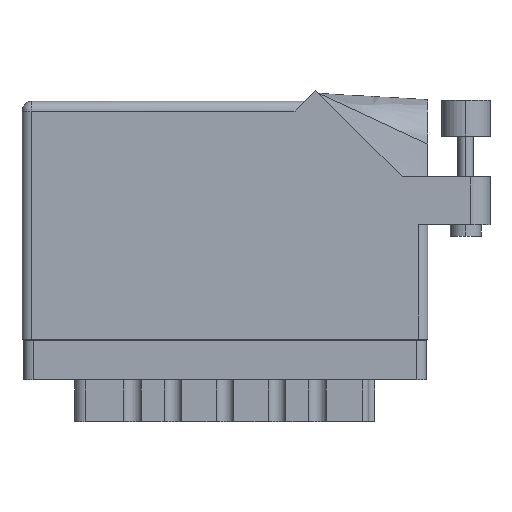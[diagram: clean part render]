
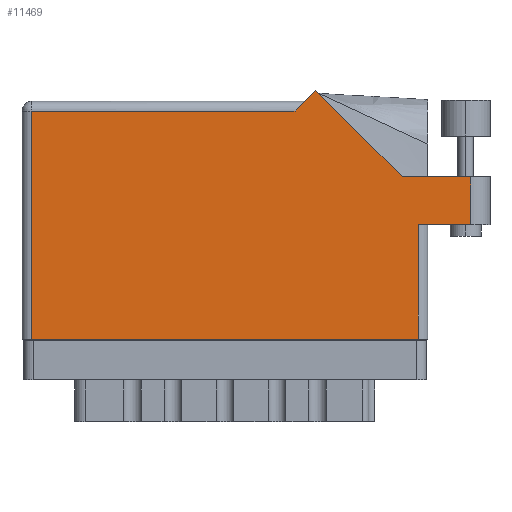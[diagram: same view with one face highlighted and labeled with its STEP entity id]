
A CAD part, front view. The second image highlights one B-rep face of the part: STEP entity #11469.
In plain terms, the highlighted face is planar.
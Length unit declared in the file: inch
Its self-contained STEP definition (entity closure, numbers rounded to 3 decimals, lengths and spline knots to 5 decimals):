
#478 = CARTESIAN_POINT ( 'NONE',  ( 2.44642, 1.044, 0. ) ) ;
#655 = VECTOR ( 'NONE', #3263, 39.37008 ) ;
#1212 = VERTEX_POINT ( 'NONE', #16223 ) ;
#1598 = CARTESIAN_POINT ( 'NONE',  ( 0., 0., 0. ) ) ;
#1919 = LINE ( 'NONE', #1598, #3772 ) ;
#3263 = DIRECTION ( 'NONE',  ( 0., 1., 0. ) ) ;
#3568 = EDGE_CURVE ( 'NONE', #42760, #24463, #35053, .T. ) ;
#3651 = VERTEX_POINT ( 'NONE', #30559 ) ;
#3772 = VECTOR ( 'NONE', #16540, 39.37008 ) ;
#4589 = ORIENTED_EDGE ( 'NONE', *, *, #44058, .T. ) ;
#7167 = VERTEX_POINT ( 'NONE', #27229 ) ;
#7701 = ORIENTED_EDGE ( 'NONE', *, *, #15196, .T. ) ;
#8189 = VERTEX_POINT ( 'NONE', #43937 ) ;
#8296 = EDGE_CURVE ( 'NONE', #1212, #13058, #34891, .T. ) ;
#8317 = VECTOR ( 'NONE', #32690, 39.37008 ) ;
#8775 = VECTOR ( 'NONE', #46525, 39.37008 ) ;
#10041 = DIRECTION ( 'NONE',  ( -1., 0., 0. ) ) ;
#11340 = CARTESIAN_POINT ( 'NONE',  ( 2.55, 0.737, 0. ) ) ;
#11469 = ADVANCED_FACE ( 'NONE', ( #12407 ), #39918, .F. ) ;
#11866 = CARTESIAN_POINT ( 'NONE',  ( 2.612, 0.737, 0. ) ) ;
#12407 = FACE_OUTER_BOUND ( 'NONE', #37761, .T. ) ;
#12431 = CARTESIAN_POINT ( 'NONE',  ( 2.887, 1.044, 0. ) ) ;
#13058 = VERTEX_POINT ( 'NONE', #25972 ) ;
#13282 = LINE ( 'NONE', #15251, #39683 ) ;
#15196 = EDGE_CURVE ( 'NONE', #34776, #42760, #1919, .T. ) ;
#15251 = CARTESIAN_POINT ( 'NONE',  ( 3.012, 1.044, 0. ) ) ;
#16223 = CARTESIAN_POINT ( 'NONE',  ( 2.44642, 1.044, 0. ) ) ;
#16485 = LINE ( 'NONE', #11866, #8775 ) ;
#16540 = DIRECTION ( 'NONE',  ( 1., 0., 0. ) ) ;
#16693 = AXIS2_PLACEMENT_3D ( 'NONE', #16948, #43768, #17430 ) ;
#16948 = CARTESIAN_POINT ( 'NONE',  ( 0., 1.53, 0. ) ) ;
#17245 = CARTESIAN_POINT ( 'NONE',  ( 0.062, 0., 0. ) ) ;
#17430 = DIRECTION ( 'NONE',  ( -1., 0., 0. ) ) ;
#17687 = ORIENTED_EDGE ( 'NONE', *, *, #29649, .T. ) ;
#18836 = VERTEX_POINT ( 'NONE', #12431 ) ;
#19114 = DIRECTION ( 'NONE',  ( -1., 0., 0. ) ) ;
#22513 = CARTESIAN_POINT ( 'NONE',  ( 2.55, 0.737, 0. ) ) ;
#23411 = VECTOR ( 'NONE', #32790, 39.37008 ) ;
#24463 = VERTEX_POINT ( 'NONE', #22513 ) ;
#24665 = VECTOR ( 'NONE', #34381, 39.37008 ) ;
#25907 = CARTESIAN_POINT ( 'NONE',  ( 2.887, 1.044, 0. ) ) ;
#25972 = CARTESIAN_POINT ( 'NONE',  ( 1.88971, 1.60071, 0. ) ) ;
#27229 = CARTESIAN_POINT ( 'NONE',  ( 1.757, 1.468, 0. ) ) ;
#27524 = EDGE_CURVE ( 'NONE', #24463, #8189, #16485, .T. ) ;
#28039 = ORIENTED_EDGE ( 'NONE', *, *, #36100, .T. ) ;
#28141 = ORIENTED_EDGE ( 'NONE', *, *, #8296, .T. ) ;
#29649 = EDGE_CURVE ( 'NONE', #18836, #1212, #13282, .T. ) ;
#30559 = CARTESIAN_POINT ( 'NONE',  ( 0.062, 1.468, 0. ) ) ;
#32690 = DIRECTION ( 'NONE',  ( 0., -1., 0. ) ) ;
#32790 = DIRECTION ( 'NONE',  ( -0.707, -0.707, 0. ) ) ;
#34381 = DIRECTION ( 'NONE',  ( -0.707, 0.707, 0. ) ) ;
#34776 = VERTEX_POINT ( 'NONE', #43867 ) ;
#34891 = LINE ( 'NONE', #478, #24665 ) ;
#35053 = LINE ( 'NONE', #11340, #36796 ) ;
#35091 = ORIENTED_EDGE ( 'NONE', *, *, #39433, .T. ) ;
#36100 = EDGE_CURVE ( 'NONE', #8189, #18836, #46086, .T. ) ;
#36796 = VECTOR ( 'NONE', #38254, 39.37008 ) ;
#37761 = EDGE_LOOP ( 'NONE', ( #45225, #28039, #17687, #28141, #37927, #35091, #4589, #7701, #47832 ) ) ;
#37927 = ORIENTED_EDGE ( 'NONE', *, *, #46476, .T. ) ;
#38254 = DIRECTION ( 'NONE',  ( 0., 1., 0. ) ) ;
#39433 = EDGE_CURVE ( 'NONE', #7167, #3651, #40406, .T. ) ;
#39683 = VECTOR ( 'NONE', #19114, 39.37008 ) ;
#39918 = PLANE ( 'NONE',  #16693 ) ;
#40406 = LINE ( 'NONE', #40868, #42828 ) ;
#40868 = CARTESIAN_POINT ( 'NONE',  ( 0., 1.468, 0. ) ) ;
#41392 = LINE ( 'NONE', #44358, #23411 ) ;
#42445 = LINE ( 'NONE', #17245, #8317 ) ;
#42760 = VERTEX_POINT ( 'NONE', #46406 ) ;
#42828 = VECTOR ( 'NONE', #10041, 39.37008 ) ;
#43768 = DIRECTION ( 'NONE',  ( 0., 0., -1. ) ) ;
#43867 = CARTESIAN_POINT ( 'NONE',  ( 0.062, 0., 0. ) ) ;
#43937 = CARTESIAN_POINT ( 'NONE',  ( 2.887, 0.737, 0. ) ) ;
#44058 = EDGE_CURVE ( 'NONE', #3651, #34776, #42445, .T. ) ;
#44358 = CARTESIAN_POINT ( 'NONE',  ( 1.819, 1.53, 0. ) ) ;
#45225 = ORIENTED_EDGE ( 'NONE', *, *, #27524, .T. ) ;
#46086 = LINE ( 'NONE', #25907, #655 ) ;
#46406 = CARTESIAN_POINT ( 'NONE',  ( 2.55, 0., 0. ) ) ;
#46476 = EDGE_CURVE ( 'NONE', #13058, #7167, #41392, .T. ) ;
#46525 = DIRECTION ( 'NONE',  ( 1., 0., 0. ) ) ;
#47832 = ORIENTED_EDGE ( 'NONE', *, *, #3568, .T. ) ;
